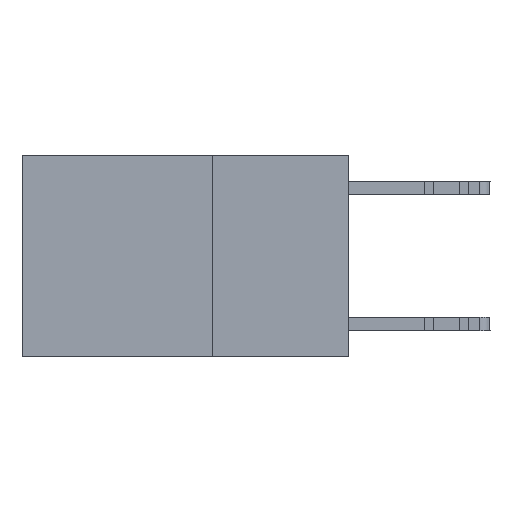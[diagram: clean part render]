
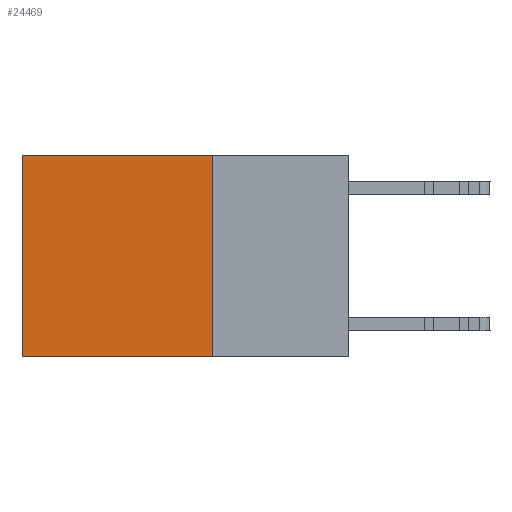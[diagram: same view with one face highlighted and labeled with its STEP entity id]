
A CAD part, left-side view. The second image highlights one B-rep face of the part: STEP entity #24469.
In plain terms, the highlighted planar face has unit normal (-1, 0, 0).
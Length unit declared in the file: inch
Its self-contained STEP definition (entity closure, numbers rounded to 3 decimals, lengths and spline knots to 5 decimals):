
#78 = AXIS2_PLACEMENT_3D ( 'NONE', #25729, #18970, #10211 ) ;
#278 = VECTOR ( 'NONE', #13670, 39.37008 ) ;
#633 = CARTESIAN_POINT ( 'NONE',  ( 0.2625, 0.6, -0.37 ) ) ;
#1675 = CARTESIAN_POINT ( 'NONE',  ( 0.2625, 0.6, 0. ) ) ;
#2114 = ORIENTED_EDGE ( 'NONE', *, *, #12504, .F. ) ;
#4145 = VERTEX_POINT ( 'NONE', #633 ) ;
#4777 = CARTESIAN_POINT ( 'NONE',  ( 0.2625, 0.25, -0.37 ) ) ;
#7151 = FACE_OUTER_BOUND ( 'NONE', #23269, .T. ) ;
#8673 = VERTEX_POINT ( 'NONE', #1675 ) ;
#9015 = LINE ( 'NONE', #4777, #278 ) ;
#9028 = DIRECTION ( 'NONE',  ( 0., 0., -1. ) ) ;
#9392 = VECTOR ( 'NONE', #9028, 39.37008 ) ;
#9780 = ORIENTED_EDGE ( 'NONE', *, *, #22120, .F. ) ;
#9883 = CARTESIAN_POINT ( 'NONE',  ( 0.2625, 0.25, 0. ) ) ;
#10211 = DIRECTION ( 'NONE',  ( 0., 0., -1. ) ) ;
#12504 = EDGE_CURVE ( 'NONE', #27272, #20705, #28142, .T. ) ;
#12717 = VECTOR ( 'NONE', #24817, 39.37008 ) ;
#13116 = LINE ( 'NONE', #26722, #12717 ) ;
#13670 = DIRECTION ( 'NONE',  ( 0., 1., 0. ) ) ;
#15307 = VECTOR ( 'NONE', #25548, 39.37008 ) ;
#15693 = ORIENTED_EDGE ( 'NONE', *, *, #24903, .T. ) ;
#15864 = LINE ( 'NONE', #18219, #9392 ) ;
#18219 = CARTESIAN_POINT ( 'NONE',  ( 0.2625, 0.6, 0. ) ) ;
#18627 = EDGE_CURVE ( 'NONE', #27272, #8673, #13116, .T. ) ;
#18970 = DIRECTION ( 'NONE',  ( 1., 0., 0. ) ) ;
#19332 = ORIENTED_EDGE ( 'NONE', *, *, #18627, .T. ) ;
#20705 = VERTEX_POINT ( 'NONE', #24045 ) ;
#20961 = CARTESIAN_POINT ( 'NONE',  ( 0.2625, 0.25, 0. ) ) ;
#21310 = PLANE ( 'NONE',  #78 ) ;
#22120 = EDGE_CURVE ( 'NONE', #20705, #4145, #9015, .T. ) ;
#23269 = EDGE_LOOP ( 'NONE', ( #15693, #9780, #2114, #19332 ) ) ;
#24045 = CARTESIAN_POINT ( 'NONE',  ( 0.2625, 0.25, -0.37 ) ) ;
#24469 = ADVANCED_FACE ( 'NONE', ( #7151 ), #21310, .F. ) ;
#24817 = DIRECTION ( 'NONE',  ( 0., 1., 0. ) ) ;
#24903 = EDGE_CURVE ( 'NONE', #8673, #4145, #15864, .T. ) ;
#25548 = DIRECTION ( 'NONE',  ( 0., 0., -1. ) ) ;
#25729 = CARTESIAN_POINT ( 'NONE',  ( 0.2625, 0.25, 0. ) ) ;
#26722 = CARTESIAN_POINT ( 'NONE',  ( 0.2625, 0.25, 0. ) ) ;
#27272 = VERTEX_POINT ( 'NONE', #20961 ) ;
#28142 = LINE ( 'NONE', #9883, #15307 ) ;
